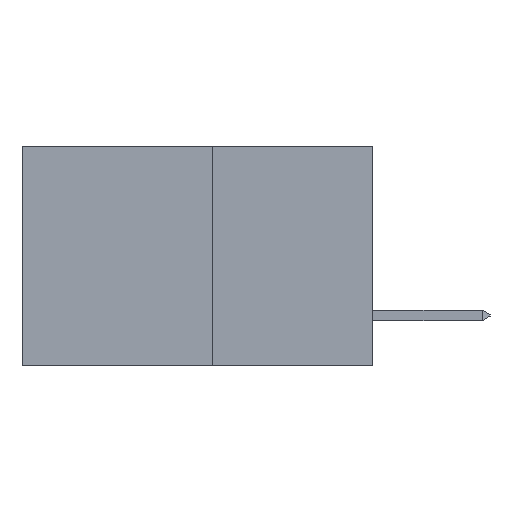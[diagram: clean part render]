
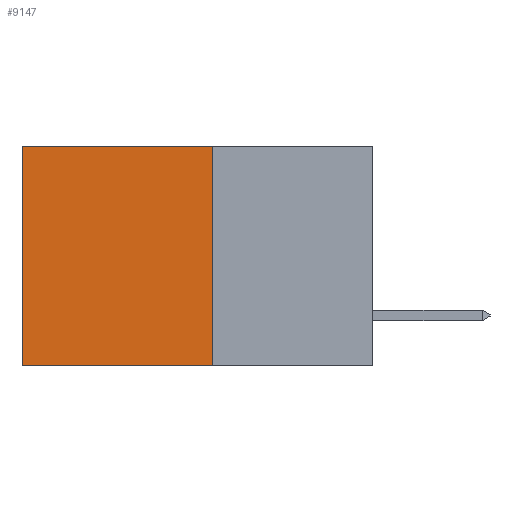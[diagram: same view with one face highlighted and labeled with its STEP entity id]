
A CAD part, left-side view. The second image highlights one B-rep face of the part: STEP entity #9147.
In plain terms, the highlighted planar face has unit normal (-1, 0, 0).
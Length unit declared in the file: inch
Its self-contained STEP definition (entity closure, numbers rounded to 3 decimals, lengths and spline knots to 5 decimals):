
#163 = LINE ( 'NONE', #4100, #8185 ) ;
#229 = ORIENTED_EDGE ( 'NONE', *, *, #7300, .T. ) ;
#246 = ORIENTED_EDGE ( 'NONE', *, *, #8063, .F. ) ;
#311 = VERTEX_POINT ( 'NONE', #6758 ) ;
#892 = LINE ( 'NONE', #1801, #8567 ) ;
#1117 = VECTOR ( 'NONE', #3811, 39.37008 ) ;
#1190 = CARTESIAN_POINT ( 'NONE',  ( 0.277, 0.59, -0.37 ) ) ;
#1248 = CARTESIAN_POINT ( 'NONE',  ( 0.277, 0.27, -0.37 ) ) ;
#1801 = CARTESIAN_POINT ( 'NONE',  ( 0.277, 0.59, -0.37 ) ) ;
#1878 = EDGE_LOOP ( 'NONE', ( #7602, #4557, #246, #229 ) ) ;
#2578 = VERTEX_POINT ( 'NONE', #6231 ) ;
#2903 = PLANE ( 'NONE',  #7491 ) ;
#2914 = DIRECTION ( 'NONE',  ( 0., 1., 0. ) ) ;
#3038 = EDGE_CURVE ( 'NONE', #2578, #4711, #163, .T. ) ;
#3682 = DIRECTION ( 'NONE',  ( 0., 0., -1. ) ) ;
#3811 = DIRECTION ( 'NONE',  ( 0., 0., -1. ) ) ;
#4100 = CARTESIAN_POINT ( 'NONE',  ( 0.277, 0.27, -0.37 ) ) ;
#4442 = CARTESIAN_POINT ( 'NONE',  ( 0.277, 0.27, 0. ) ) ;
#4557 = ORIENTED_EDGE ( 'NONE', *, *, #3038, .F. ) ;
#4711 = VERTEX_POINT ( 'NONE', #1190 ) ;
#6007 = VERTEX_POINT ( 'NONE', #9577 ) ;
#6231 = CARTESIAN_POINT ( 'NONE',  ( 0.277, 0.27, -0.37 ) ) ;
#6439 = VECTOR ( 'NONE', #2914, 39.37008 ) ;
#6758 = CARTESIAN_POINT ( 'NONE',  ( 0.277, 0.27, 0. ) ) ;
#7098 = LINE ( 'NONE', #8265, #1117 ) ;
#7300 = EDGE_CURVE ( 'NONE', #311, #6007, #8331, .T. ) ;
#7491 = AXIS2_PLACEMENT_3D ( 'NONE', #1248, #8171, #3682 ) ;
#7565 = DIRECTION ( 'NONE',  ( 0., 1., 0. ) ) ;
#7602 = ORIENTED_EDGE ( 'NONE', *, *, #8895, .T. ) ;
#7925 = DIRECTION ( 'NONE',  ( 0., 0., -1. ) ) ;
#8063 = EDGE_CURVE ( 'NONE', #311, #2578, #7098, .T. ) ;
#8171 = DIRECTION ( 'NONE',  ( 1., 0., 0. ) ) ;
#8185 = VECTOR ( 'NONE', #7565, 39.37008 ) ;
#8265 = CARTESIAN_POINT ( 'NONE',  ( 0.277, 0.27, -0.37 ) ) ;
#8331 = LINE ( 'NONE', #4442, #6439 ) ;
#8454 = FACE_OUTER_BOUND ( 'NONE', #1878, .T. ) ;
#8567 = VECTOR ( 'NONE', #7925, 39.37008 ) ;
#8895 = EDGE_CURVE ( 'NONE', #6007, #4711, #892, .T. ) ;
#9147 = ADVANCED_FACE ( 'NONE', ( #8454 ), #2903, .F. ) ;
#9577 = CARTESIAN_POINT ( 'NONE',  ( 0.277, 0.59, 0. ) ) ;
